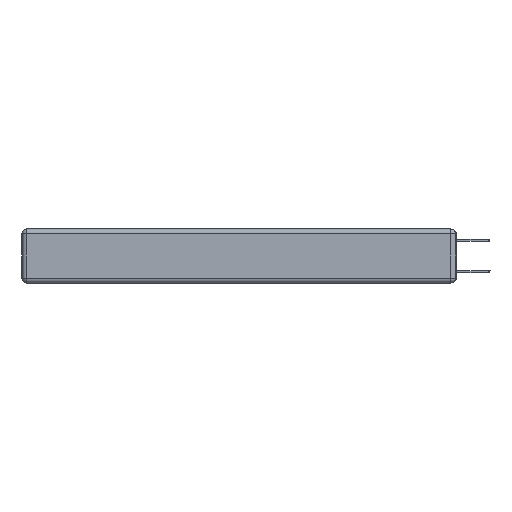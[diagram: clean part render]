
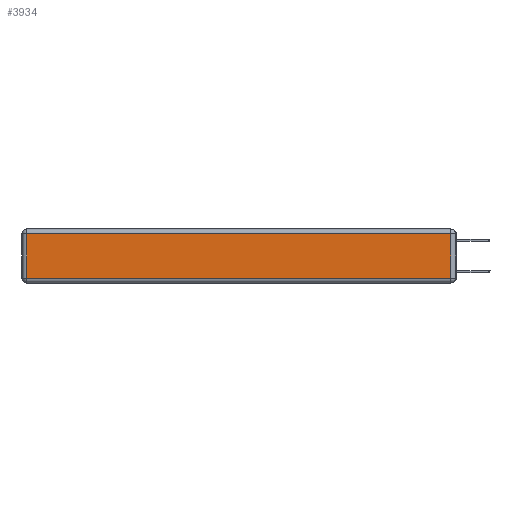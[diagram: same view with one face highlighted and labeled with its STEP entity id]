
A CAD part, left-side view. The second image highlights one B-rep face of the part: STEP entity #3934.
In plain terms, the highlighted planar face has unit normal (-1, 0, 0).
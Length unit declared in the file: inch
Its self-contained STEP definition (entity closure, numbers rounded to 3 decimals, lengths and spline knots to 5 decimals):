
#287 = VERTEX_POINT ( 'NONE', #11982 ) ;
#353 = DIRECTION ( 'NONE',  ( 0., 0., -1. ) ) ;
#564 = AXIS2_PLACEMENT_3D ( 'NONE', #14073, #18616, #2154 ) ;
#744 = EDGE_CURVE ( 'NONE', #4986, #17307, #4701, .T. ) ;
#1450 = EDGE_LOOP ( 'NONE', ( #2193, #7159, #12578, #3994 ) ) ;
#1786 = VERTEX_POINT ( 'NONE', #3403 ) ;
#2096 = PLANE ( 'NONE',  #564 ) ;
#2154 = DIRECTION ( 'NONE',  ( 0., 0., 1. ) ) ;
#2193 = ORIENTED_EDGE ( 'NONE', *, *, #744, .T. ) ;
#2932 = EDGE_CURVE ( 'NONE', #17307, #1786, #18195, .T. ) ;
#3403 = CARTESIAN_POINT ( 'NONE',  ( 0., 0.03, -0.03 ) ) ;
#3934 = ADVANCED_FACE ( 'NONE', ( #11816 ), #2096, .T. ) ;
#3994 = ORIENTED_EDGE ( 'NONE', *, *, #4620, .T. ) ;
#4620 = EDGE_CURVE ( 'NONE', #287, #4986, #10374, .T. ) ;
#4701 = LINE ( 'NONE', #11830, #13598 ) ;
#4986 = VERTEX_POINT ( 'NONE', #13089 ) ;
#6918 = DIRECTION ( 'NONE',  ( 0., 0., 1. ) ) ;
#7159 = ORIENTED_EDGE ( 'NONE', *, *, #2932, .T. ) ;
#7833 = CARTESIAN_POINT ( 'NONE',  ( 0., 2.75, -0.03 ) ) ;
#9646 = CARTESIAN_POINT ( 'NONE',  ( 0., 0.03, -0.313 ) ) ;
#9726 = VECTOR ( 'NONE', #13646, 39.37008 ) ;
#9897 = VECTOR ( 'NONE', #353, 39.37008 ) ;
#9954 = CARTESIAN_POINT ( 'NONE',  ( 0., 0.03, -0.343 ) ) ;
#10374 = LINE ( 'NONE', #10697, #9897 ) ;
#10697 = CARTESIAN_POINT ( 'NONE',  ( 0., 2.72, -0.343 ) ) ;
#11816 = FACE_OUTER_BOUND ( 'NONE', #1450, .T. ) ;
#11830 = CARTESIAN_POINT ( 'NONE',  ( 0., 0., -0.313 ) ) ;
#11982 = CARTESIAN_POINT ( 'NONE',  ( 0., 2.72, -0.03 ) ) ;
#12316 = EDGE_CURVE ( 'NONE', #1786, #287, #18424, .T. ) ;
#12578 = ORIENTED_EDGE ( 'NONE', *, *, #12316, .T. ) ;
#13089 = CARTESIAN_POINT ( 'NONE',  ( 0., 2.72, -0.313 ) ) ;
#13598 = VECTOR ( 'NONE', #14564, 39.37008 ) ;
#13646 = DIRECTION ( 'NONE',  ( 0., 1., 0. ) ) ;
#14073 = CARTESIAN_POINT ( 'NONE',  ( 0., 0., -0.343 ) ) ;
#14564 = DIRECTION ( 'NONE',  ( 0., -1., 0. ) ) ;
#17307 = VERTEX_POINT ( 'NONE', #9646 ) ;
#17960 = VECTOR ( 'NONE', #6918, 39.37008 ) ;
#18195 = LINE ( 'NONE', #9954, #17960 ) ;
#18424 = LINE ( 'NONE', #7833, #9726 ) ;
#18616 = DIRECTION ( 'NONE',  ( -1., 0., 0. ) ) ;
